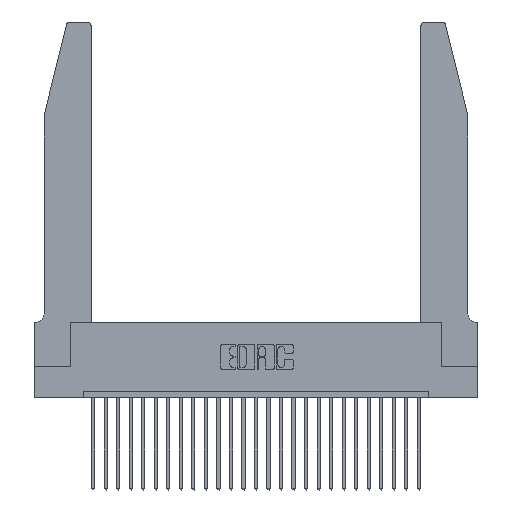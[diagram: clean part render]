
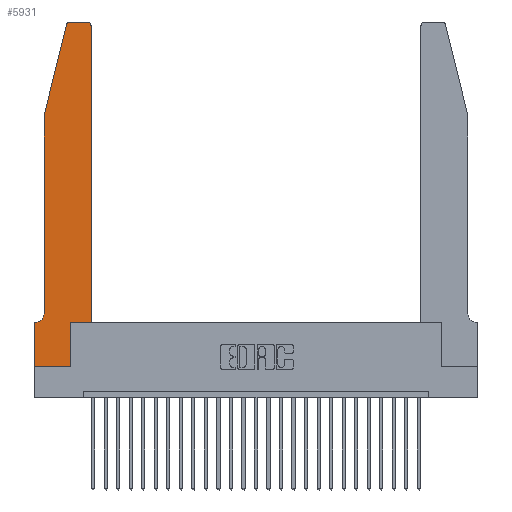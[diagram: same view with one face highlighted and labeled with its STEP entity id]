
A CAD part, top view. The second image highlights one B-rep face of the part: STEP entity #5931.
In plain terms, the highlighted planar face has unit normal (0, 0, 1).
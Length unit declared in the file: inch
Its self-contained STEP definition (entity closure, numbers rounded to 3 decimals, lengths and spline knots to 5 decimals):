
#412 = VERTEX_POINT ( 'NONE', #558 ) ;
#533 = DIRECTION ( 'NONE',  ( 0., 0., -1. ) ) ;
#558 = CARTESIAN_POINT ( 'NONE',  ( 0.2865, 0.35, 0.37 ) ) ;
#980 = VERTEX_POINT ( 'NONE', #25581 ) ;
#1161 = EDGE_CURVE ( 'NONE', #980, #10474, #18802, .T. ) ;
#1526 = DIRECTION ( 'NONE',  ( -1., 0., 0. ) ) ;
#1583 = VERTEX_POINT ( 'NONE', #10849 ) ;
#1659 = CIRCLE ( 'NONE', #15866, 0.03 ) ;
#1722 = CARTESIAN_POINT ( 'NONE',  ( 0.0755, 2., 0.37 ) ) ;
#2012 = VERTEX_POINT ( 'NONE', #9775 ) ;
#2313 = ORIENTED_EDGE ( 'NONE', *, *, #8665, .T. ) ;
#2383 = LINE ( 'NONE', #19104, #15350 ) ;
#2612 = ORIENTED_EDGE ( 'NONE', *, *, #23373, .T. ) ;
#2633 = DIRECTION ( 'NONE',  ( -1., 0., 0. ) ) ;
#2658 = CIRCLE ( 'NONE', #14086, 0.07 ) ;
#2871 = CARTESIAN_POINT ( 'NONE',  ( 0.4505, 0.35, 0.37 ) ) ;
#3095 = VECTOR ( 'NONE', #13204, 39.37008 ) ;
#3633 = ORIENTED_EDGE ( 'NONE', *, *, #7092, .T. ) ;
#4147 = EDGE_CURVE ( 'NONE', #4171, #9714, #2383, .T. ) ;
#4171 = VERTEX_POINT ( 'NONE', #25485 ) ;
#4430 = PLANE ( 'NONE',  #14011 ) ;
#4593 = EDGE_LOOP ( 'NONE', ( #17654, #9269, #2313, #19633, #22390, #2612, #18596, #23716, #3633, #21415, #14484, #12659 ) ) ;
#4897 = CARTESIAN_POINT ( 'NONE',  ( 0., 0., 0.37 ) ) ;
#4976 = VERTEX_POINT ( 'NONE', #6247 ) ;
#5034 = DIRECTION ( 'NONE',  ( 0., 0., 1. ) ) ;
#5055 = LINE ( 'NONE', #15343, #8016 ) ;
#5530 = EDGE_CURVE ( 'NONE', #1583, #13020, #10418, .T. ) ;
#5931 = ADVANCED_FACE ( 'NONE', ( #22857 ), #4430, .T. ) ;
#6036 = DIRECTION ( 'NONE',  ( -0.239, -0.971, 0. ) ) ;
#6247 = CARTESIAN_POINT ( 'NONE',  ( 0.284, 2.75, 0.37 ) ) ;
#6555 = CARTESIAN_POINT ( 'NONE',  ( 0., 0.35, 0.37 ) ) ;
#6865 = DIRECTION ( 'NONE',  ( 1., 0., 0. ) ) ;
#6931 = CARTESIAN_POINT ( 'NONE',  ( 0.284, 2.72, 0.37 ) ) ;
#7001 = LINE ( 'NONE', #22404, #16153 ) ;
#7092 = EDGE_CURVE ( 'NONE', #2012, #412, #20270, .T. ) ;
#8016 = VECTOR ( 'NONE', #6865, 39.37008 ) ;
#8654 = DIRECTION ( 'NONE',  ( 1., 0., 0. ) ) ;
#8657 = DIRECTION ( 'NONE',  ( 0., -1., 0. ) ) ;
#8665 = EDGE_CURVE ( 'NONE', #21391, #1583, #14303, .T. ) ;
#8973 = VECTOR ( 'NONE', #21812, 39.37008 ) ;
#9269 = ORIENTED_EDGE ( 'NONE', *, *, #15344, .T. ) ;
#9428 = CARTESIAN_POINT ( 'NONE',  ( 0.25487, 2.72718, 0.37 ) ) ;
#9714 = VERTEX_POINT ( 'NONE', #9842 ) ;
#9775 = CARTESIAN_POINT ( 'NONE',  ( 0.2865, 0., 0.37 ) ) ;
#9842 = CARTESIAN_POINT ( 'NONE',  ( 0., 0., 0.37 ) ) ;
#10117 = EDGE_CURVE ( 'NONE', #9714, #2012, #21113, .T. ) ;
#10418 = LINE ( 'NONE', #10668, #12351 ) ;
#10474 = VERTEX_POINT ( 'NONE', #24912 ) ;
#10475 = EDGE_CURVE ( 'NONE', #412, #980, #5055, .T. ) ;
#10668 = CARTESIAN_POINT ( 'NONE',  ( 0.0755, 2., 0.37 ) ) ;
#10849 = CARTESIAN_POINT ( 'NONE',  ( 0.0755, 2., 0.37 ) ) ;
#12054 = EDGE_CURVE ( 'NONE', #13020, #26819, #2658, .T. ) ;
#12351 = VECTOR ( 'NONE', #21235, 39.37008 ) ;
#12422 = DIRECTION ( 'NONE',  ( 0., 1., 0. ) ) ;
#12659 = ORIENTED_EDGE ( 'NONE', *, *, #14175, .T. ) ;
#13020 = VERTEX_POINT ( 'NONE', #22714 ) ;
#13204 = DIRECTION ( 'NONE',  ( 1., 0., 0. ) ) ;
#13218 = DIRECTION ( 'NONE',  ( 0., 0., 1. ) ) ;
#13518 = DIRECTION ( 'NONE',  ( 1., 0., 0. ) ) ;
#14011 = AXIS2_PLACEMENT_3D ( 'NONE', #6555, #21173, #8654 ) ;
#14086 = AXIS2_PLACEMENT_3D ( 'NONE', #19502, #533, #2633 ) ;
#14175 = EDGE_CURVE ( 'NONE', #10474, #24924, #14471, .T. ) ;
#14303 = LINE ( 'NONE', #1722, #18583 ) ;
#14471 = CIRCLE ( 'NONE', #17441, 0.03 ) ;
#14484 = ORIENTED_EDGE ( 'NONE', *, *, #1161, .T. ) ;
#15343 = CARTESIAN_POINT ( 'NONE',  ( 0.4505, 0.35, 0.37 ) ) ;
#15344 = EDGE_CURVE ( 'NONE', #4976, #21391, #1659, .T. ) ;
#15350 = VECTOR ( 'NONE', #8657, 39.37008 ) ;
#15866 = AXIS2_PLACEMENT_3D ( 'NONE', #6931, #13218, #21732 ) ;
#16021 = VECTOR ( 'NONE', #12422, 39.37008 ) ;
#16153 = VECTOR ( 'NONE', #1526, 39.37008 ) ;
#17441 = AXIS2_PLACEMENT_3D ( 'NONE', #24108, #5034, #13518 ) ;
#17654 = ORIENTED_EDGE ( 'NONE', *, *, #21485, .T. ) ;
#18483 = CARTESIAN_POINT ( 'NONE',  ( 0.0055, 0.35, 0.37 ) ) ;
#18583 = VECTOR ( 'NONE', #6036, 39.37008 ) ;
#18596 = ORIENTED_EDGE ( 'NONE', *, *, #4147, .T. ) ;
#18802 = LINE ( 'NONE', #2871, #8973 ) ;
#19104 = CARTESIAN_POINT ( 'NONE',  ( 0., 0., 0.37 ) ) ;
#19199 = CARTESIAN_POINT ( 'NONE',  ( 0.0755, 0.35, 0.37 ) ) ;
#19502 = CARTESIAN_POINT ( 'NONE',  ( 0.0055, 0.42, 0.37 ) ) ;
#19633 = ORIENTED_EDGE ( 'NONE', *, *, #5530, .T. ) ;
#20270 = LINE ( 'NONE', #22924, #16021 ) ;
#21113 = LINE ( 'NONE', #4897, #3095 ) ;
#21173 = DIRECTION ( 'NONE',  ( 0., 0., 1. ) ) ;
#21235 = DIRECTION ( 'NONE',  ( 0., -1., 0. ) ) ;
#21266 = DIRECTION ( 'NONE',  ( -1., 0., 0. ) ) ;
#21391 = VERTEX_POINT ( 'NONE', #9428 ) ;
#21415 = ORIENTED_EDGE ( 'NONE', *, *, #10475, .T. ) ;
#21485 = EDGE_CURVE ( 'NONE', #24924, #4976, #7001, .T. ) ;
#21732 = DIRECTION ( 'NONE',  ( 1., 0., 0. ) ) ;
#21812 = DIRECTION ( 'NONE',  ( 0., 1., 0. ) ) ;
#22390 = ORIENTED_EDGE ( 'NONE', *, *, #12054, .T. ) ;
#22404 = CARTESIAN_POINT ( 'NONE',  ( 0.2605, 2.75, 0.37 ) ) ;
#22714 = CARTESIAN_POINT ( 'NONE',  ( 0.0755, 0.42, 0.37 ) ) ;
#22857 = FACE_OUTER_BOUND ( 'NONE', #4593, .T. ) ;
#22924 = CARTESIAN_POINT ( 'NONE',  ( 0.2865, 0.35, 0.37 ) ) ;
#23373 = EDGE_CURVE ( 'NONE', #26819, #4171, #24640, .T. ) ;
#23660 = VECTOR ( 'NONE', #21266, 39.37008 ) ;
#23716 = ORIENTED_EDGE ( 'NONE', *, *, #10117, .T. ) ;
#24108 = CARTESIAN_POINT ( 'NONE',  ( 0.4205, 2.72, 0.37 ) ) ;
#24640 = LINE ( 'NONE', #19199, #23660 ) ;
#24912 = CARTESIAN_POINT ( 'NONE',  ( 0.4505, 2.72, 0.37 ) ) ;
#24924 = VERTEX_POINT ( 'NONE', #26214 ) ;
#25485 = CARTESIAN_POINT ( 'NONE',  ( 0., 0.35, 0.37 ) ) ;
#25581 = CARTESIAN_POINT ( 'NONE',  ( 0.4505, 0.35, 0.37 ) ) ;
#26214 = CARTESIAN_POINT ( 'NONE',  ( 0.4205, 2.75, 0.37 ) ) ;
#26819 = VERTEX_POINT ( 'NONE', #18483 ) ;
